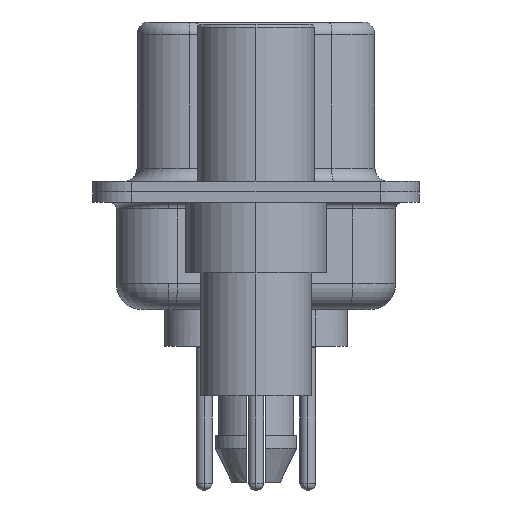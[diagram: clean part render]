
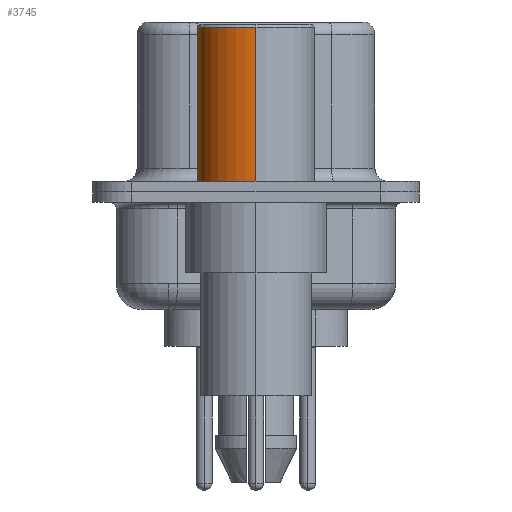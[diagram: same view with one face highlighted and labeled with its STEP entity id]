
A CAD part, left-side view. The second image highlights one B-rep face of the part: STEP entity #3745.
In plain terms, the highlighted cylindrical face has radius 2.25 mm (diameter 4.5 mm), a partial arc.
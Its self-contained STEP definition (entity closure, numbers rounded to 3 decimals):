
#61 = CARTESIAN_POINT ( 'NONE',  ( 2.25, 0., 0.4 ) ) ;
#326 = CARTESIAN_POINT ( 'NONE',  ( 0., 0., 0.4 ) ) ;
#1088 = DIRECTION ( 'NONE',  ( 0., 0., 1. ) ) ;
#1242 = CARTESIAN_POINT ( 'NONE',  ( 2.25, 0., 0.581 ) ) ;
#1715 = AXIS2_PLACEMENT_3D ( 'NONE', #10485, #25109, #12611 ) ;
#2457 = EDGE_CURVE ( 'NONE', #15488, #15725, #20779, .T. ) ;
#2575 = DIRECTION ( 'NONE',  ( 1., 0., 0. ) ) ;
#3395 = ORIENTED_EDGE ( 'NONE', *, *, #2457, .T. ) ;
#3745 = ADVANCED_FACE ( 'NONE', ( #23023 ), #6246, .T. ) ;
#5237 = EDGE_CURVE ( 'NONE', #26287, #17092, #15112, .T. ) ;
#6246 = CYLINDRICAL_SURFACE ( 'NONE', #26858, 2.25 ) ;
#8060 = ORIENTED_EDGE ( 'NONE', *, *, #22619, .T. ) ;
#9285 = ORIENTED_EDGE ( 'NONE', *, *, #11026, .F. ) ;
#9505 = VECTOR ( 'NONE', #1088, 1000. ) ;
#9649 = CIRCLE ( 'NONE', #1715, 2.25 ) ;
#10175 = CARTESIAN_POINT ( 'NONE',  ( 0., 0., 0.581 ) ) ;
#10485 = CARTESIAN_POINT ( 'NONE',  ( 0., 0., 6.3 ) ) ;
#11026 = EDGE_CURVE ( 'NONE', #17092, #15725, #9649, .T. ) ;
#11377 = DIRECTION ( 'NONE',  ( 0., 0., 1. ) ) ;
#12019 = CARTESIAN_POINT ( 'NONE',  ( -2.25, 0., 0.581 ) ) ;
#12266 = CARTESIAN_POINT ( 'NONE',  ( -2.25, 0., 0.4 ) ) ;
#12611 = DIRECTION ( 'NONE',  ( 1., 0., 0. ) ) ;
#13327 = CIRCLE ( 'NONE', #13465, 2.25 ) ;
#13465 = AXIS2_PLACEMENT_3D ( 'NONE', #326, #15323, #2575 ) ;
#15070 = ORIENTED_EDGE ( 'NONE', *, *, #5237, .F. ) ;
#15112 = LINE ( 'NONE', #1242, #9505 ) ;
#15231 = VECTOR ( 'NONE', #11377, 1000. ) ;
#15323 = DIRECTION ( 'NONE',  ( 0., 0., 1. ) ) ;
#15488 = VERTEX_POINT ( 'NONE', #12266 ) ;
#15725 = VERTEX_POINT ( 'NONE', #21452 ) ;
#17092 = VERTEX_POINT ( 'NONE', #17933 ) ;
#17933 = CARTESIAN_POINT ( 'NONE',  ( 2.25, 0., 6.3 ) ) ;
#20779 = LINE ( 'NONE', #12019, #15231 ) ;
#21452 = CARTESIAN_POINT ( 'NONE',  ( -2.25, 0., 6.3 ) ) ;
#22619 = EDGE_CURVE ( 'NONE', #26287, #15488, #13327, .T. ) ;
#23023 = FACE_OUTER_BOUND ( 'NONE', #23136, .T. ) ;
#23136 = EDGE_LOOP ( 'NONE', ( #8060, #3395, #9285, #15070 ) ) ;
#23228 = DIRECTION ( 'NONE',  ( 1., 0., 0. ) ) ;
#25008 = DIRECTION ( 'NONE',  ( 0., 0., 1. ) ) ;
#25109 = DIRECTION ( 'NONE',  ( 0., 0., 1. ) ) ;
#26287 = VERTEX_POINT ( 'NONE', #61 ) ;
#26858 = AXIS2_PLACEMENT_3D ( 'NONE', #10175, #25008, #23228 ) ;
